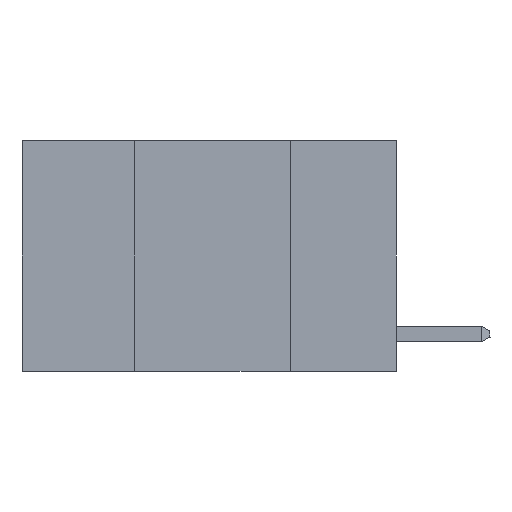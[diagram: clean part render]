
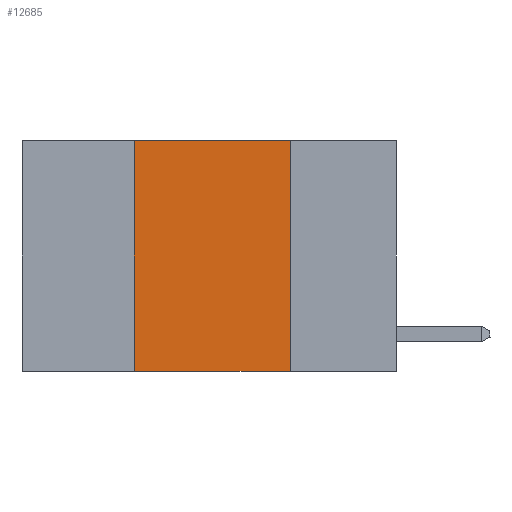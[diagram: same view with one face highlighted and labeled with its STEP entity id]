
A CAD part, left-side view. The second image highlights one B-rep face of the part: STEP entity #12685.
In plain terms, the highlighted planar face has unit normal (-1, 0, 0).
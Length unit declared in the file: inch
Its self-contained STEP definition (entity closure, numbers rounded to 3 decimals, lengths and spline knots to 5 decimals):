
#233 = ORIENTED_EDGE ( 'NONE', *, *, #1898, .F. ) ;
#265 = CARTESIAN_POINT ( 'NONE',  ( 0., 0.42, -0.37 ) ) ;
#267 = AXIS2_PLACEMENT_3D ( 'NONE', #8768, #8997, #4117 ) ;
#528 = VERTEX_POINT ( 'NONE', #10804 ) ;
#775 = EDGE_LOOP ( 'NONE', ( #1394, #233, #5844, #14208 ) ) ;
#1296 = VECTOR ( 'NONE', #11383, 39.37008 ) ;
#1394 = ORIENTED_EDGE ( 'NONE', *, *, #5916, .F. ) ;
#1898 = EDGE_CURVE ( 'NONE', #12578, #14607, #6756, .T. ) ;
#2783 = EDGE_CURVE ( 'NONE', #6062, #528, #8005, .T. ) ;
#3579 = CARTESIAN_POINT ( 'NONE',  ( 0., 0.42, 0. ) ) ;
#4117 = DIRECTION ( 'NONE',  ( 0., 0., -1. ) ) ;
#4323 = CARTESIAN_POINT ( 'NONE',  ( 0., 0.17, 0. ) ) ;
#4415 = PLANE ( 'NONE',  #267 ) ;
#4935 = VECTOR ( 'NONE', #8894, 39.37008 ) ;
#5844 = ORIENTED_EDGE ( 'NONE', *, *, #13949, .F. ) ;
#5916 = EDGE_CURVE ( 'NONE', #14607, #528, #10397, .T. ) ;
#6062 = VERTEX_POINT ( 'NONE', #265 ) ;
#6499 = CARTESIAN_POINT ( 'NONE',  ( 0., 0.42, 0. ) ) ;
#6577 = FACE_OUTER_BOUND ( 'NONE', #775, .T. ) ;
#6756 = LINE ( 'NONE', #14617, #11560 ) ;
#7485 = CARTESIAN_POINT ( 'NONE',  ( 0., 0.17, 0. ) ) ;
#8005 = LINE ( 'NONE', #12580, #1296 ) ;
#8586 = VECTOR ( 'NONE', #12697, 39.37008 ) ;
#8768 = CARTESIAN_POINT ( 'NONE',  ( 0., 0.6, 0. ) ) ;
#8878 = DIRECTION ( 'NONE',  ( 0., -1., 0. ) ) ;
#8894 = DIRECTION ( 'NONE',  ( 0., 0., -1. ) ) ;
#8997 = DIRECTION ( 'NONE',  ( 1., 0., 0. ) ) ;
#10397 = LINE ( 'NONE', #4323, #4935 ) ;
#10602 = LINE ( 'NONE', #3579, #8586 ) ;
#10804 = CARTESIAN_POINT ( 'NONE',  ( 0., 0.17, -0.37 ) ) ;
#11383 = DIRECTION ( 'NONE',  ( 0., -1., 0. ) ) ;
#11560 = VECTOR ( 'NONE', #8878, 39.37008 ) ;
#12578 = VERTEX_POINT ( 'NONE', #6499 ) ;
#12580 = CARTESIAN_POINT ( 'NONE',  ( 0., 0.6, -0.37 ) ) ;
#12685 = ADVANCED_FACE ( 'NONE', ( #6577 ), #4415, .F. ) ;
#12697 = DIRECTION ( 'NONE',  ( 0., 0., 1. ) ) ;
#13949 = EDGE_CURVE ( 'NONE', #6062, #12578, #10602, .T. ) ;
#14208 = ORIENTED_EDGE ( 'NONE', *, *, #2783, .T. ) ;
#14607 = VERTEX_POINT ( 'NONE', #7485 ) ;
#14617 = CARTESIAN_POINT ( 'NONE',  ( 0., 0.6, 0. ) ) ;
